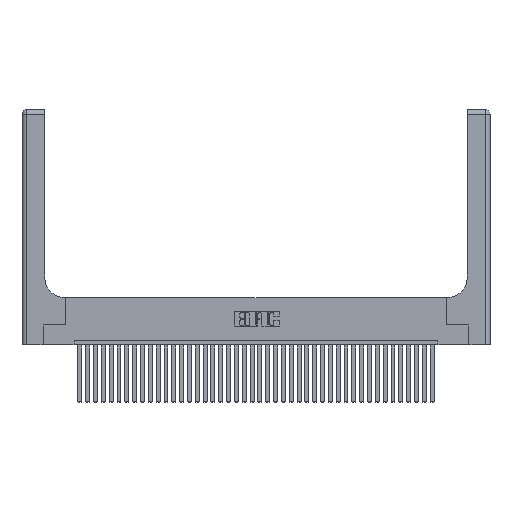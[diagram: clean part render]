
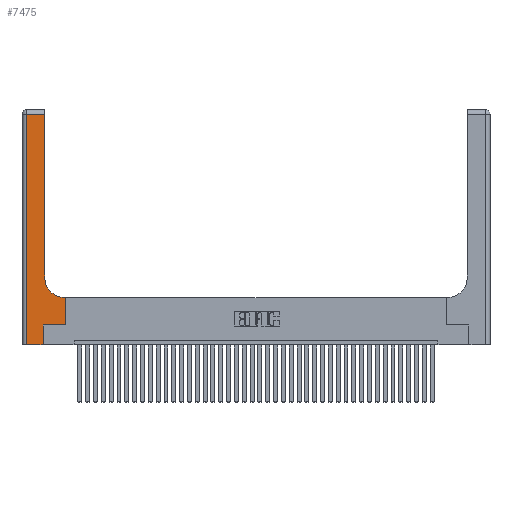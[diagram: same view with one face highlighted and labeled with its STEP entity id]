
A CAD part, top view. The second image highlights one B-rep face of the part: STEP entity #7475.
In plain terms, the highlighted planar face has unit normal (0, 0, 1).
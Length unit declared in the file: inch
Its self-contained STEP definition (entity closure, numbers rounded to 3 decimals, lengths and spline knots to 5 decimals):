
#110 = VECTOR ( 'NONE', #11667, 39.37008 ) ;
#833 = VECTOR ( 'NONE', #35096, 39.37008 ) ;
#1074 = LINE ( 'NONE', #33488, #17229 ) ;
#1376 = DIRECTION ( 'NONE',  ( -1., 0., 0. ) ) ;
#1617 = CARTESIAN_POINT ( 'NONE',  ( 0.06, 0., 0.37 ) ) ;
#1853 = LINE ( 'NONE', #7689, #833 ) ;
#2004 = ORIENTED_EDGE ( 'NONE', *, *, #32239, .T. ) ;
#2852 = ORIENTED_EDGE ( 'NONE', *, *, #15373, .T. ) ;
#4505 = DIRECTION ( 'NONE',  ( -1., 0., 0. ) ) ;
#5260 = CARTESIAN_POINT ( 'NONE',  ( 0.2915, 0.85, 0.37 ) ) ;
#5658 = EDGE_LOOP ( 'NONE', ( #2852, #28928, #32468, #20395, #30731, #34978, #31533, #2004, #23931 ) ) ;
#5990 = VERTEX_POINT ( 'NONE', #32573 ) ;
#6910 = DIRECTION ( 'NONE',  ( -1., 0., 0. ) ) ;
#7069 = DIRECTION ( 'NONE',  ( 0., 0., -1. ) ) ;
#7203 = PLANE ( 'NONE',  #17734 ) ;
#7336 = VECTOR ( 'NONE', #6910, 39.37008 ) ;
#7390 = LINE ( 'NONE', #30518, #8805 ) ;
#7475 = ADVANCED_FACE ( 'NONE', ( #32360 ), #7203, .F. ) ;
#7689 = CARTESIAN_POINT ( 'NONE',  ( 0., 0., 0.37 ) ) ;
#8541 = EDGE_CURVE ( 'NONE', #35773, #21670, #36857, .T. ) ;
#8805 = VECTOR ( 'NONE', #9416, 39.37008 ) ;
#9416 = DIRECTION ( 'NONE',  ( 0., 1., 0. ) ) ;
#10123 = VERTEX_POINT ( 'NONE', #34058 ) ;
#11398 = AXIS2_PLACEMENT_3D ( 'NONE', #24313, #18217, #30767 ) ;
#11667 = DIRECTION ( 'NONE',  ( 0., 1., 0. ) ) ;
#12252 = VERTEX_POINT ( 'NONE', #33905 ) ;
#13229 = EDGE_CURVE ( 'NONE', #32001, #12252, #24345, .T. ) ;
#13481 = CARTESIAN_POINT ( 'NONE',  ( 0.2915, 0.6, 0.37 ) ) ;
#15198 = DIRECTION ( 'NONE',  ( 0., -1., 0. ) ) ;
#15335 = CARTESIAN_POINT ( 'NONE',  ( 0.2915, 2.94, 0.37 ) ) ;
#15373 = EDGE_CURVE ( 'NONE', #31047, #32001, #35571, .T. ) ;
#15817 = CARTESIAN_POINT ( 'NONE',  ( 0.2915, 3., 0.37 ) ) ;
#17229 = VECTOR ( 'NONE', #15198, 39.37008 ) ;
#17597 = EDGE_CURVE ( 'NONE', #5990, #31047, #22143, .T. ) ;
#17734 = AXIS2_PLACEMENT_3D ( 'NONE', #22519, #7069, #1376 ) ;
#17858 = VERTEX_POINT ( 'NONE', #29990 ) ;
#18140 = CARTESIAN_POINT ( 'NONE',  ( 0., 2.94, 0.37 ) ) ;
#18217 = DIRECTION ( 'NONE',  ( 0., 0., -1. ) ) ;
#18834 = DIRECTION ( 'NONE',  ( 0., 1., 0. ) ) ;
#20100 = VERTEX_POINT ( 'NONE', #1617 ) ;
#20306 = EDGE_CURVE ( 'NONE', #21670, #10123, #37862, .T. ) ;
#20395 = ORIENTED_EDGE ( 'NONE', *, *, #34168, .T. ) ;
#21670 = VERTEX_POINT ( 'NONE', #34632 ) ;
#21705 = CARTESIAN_POINT ( 'NONE',  ( 0.269, 0.25, 0.37 ) ) ;
#22143 = CIRCLE ( 'NONE', #11398, 0.25 ) ;
#22519 = CARTESIAN_POINT ( 'NONE',  ( 0., 3., 0.37 ) ) ;
#23104 = DIRECTION ( 'NONE',  ( 1., 0., 0. ) ) ;
#23931 = ORIENTED_EDGE ( 'NONE', *, *, #17597, .T. ) ;
#24313 = CARTESIAN_POINT ( 'NONE',  ( 0.5415, 0.85, 0.37 ) ) ;
#24345 = LINE ( 'NONE', #18140, #7336 ) ;
#24432 = EDGE_CURVE ( 'NONE', #17858, #35773, #7390, .T. ) ;
#28928 = ORIENTED_EDGE ( 'NONE', *, *, #13229, .T. ) ;
#29246 = LINE ( 'NONE', #13481, #37620 ) ;
#29990 = CARTESIAN_POINT ( 'NONE',  ( 0.269, 0., 0.37 ) ) ;
#30131 = CARTESIAN_POINT ( 'NONE',  ( 0.5585, 0.25, 0.37 ) ) ;
#30518 = CARTESIAN_POINT ( 'NONE',  ( 0.269, 0., 0.37 ) ) ;
#30731 = ORIENTED_EDGE ( 'NONE', *, *, #24432, .T. ) ;
#30767 = DIRECTION ( 'NONE',  ( 1., 0., 0. ) ) ;
#31047 = VERTEX_POINT ( 'NONE', #5260 ) ;
#31533 = ORIENTED_EDGE ( 'NONE', *, *, #20306, .T. ) ;
#32001 = VERTEX_POINT ( 'NONE', #15335 ) ;
#32239 = EDGE_CURVE ( 'NONE', #10123, #5990, #29246, .T. ) ;
#32360 = FACE_OUTER_BOUND ( 'NONE', #5658, .T. ) ;
#32468 = ORIENTED_EDGE ( 'NONE', *, *, #36963, .T. ) ;
#32484 = CARTESIAN_POINT ( 'NONE',  ( 0.269, 0.25, 0.37 ) ) ;
#32573 = CARTESIAN_POINT ( 'NONE',  ( 0.5415, 0.6, 0.37 ) ) ;
#33488 = CARTESIAN_POINT ( 'NONE',  ( 0.06, 3., 0.37 ) ) ;
#33905 = CARTESIAN_POINT ( 'NONE',  ( 0.06, 2.94, 0.37 ) ) ;
#34058 = CARTESIAN_POINT ( 'NONE',  ( 0.5585, 0.6, 0.37 ) ) ;
#34168 = EDGE_CURVE ( 'NONE', #20100, #17858, #1853, .T. ) ;
#34632 = CARTESIAN_POINT ( 'NONE',  ( 0.5585, 0.25, 0.37 ) ) ;
#34978 = ORIENTED_EDGE ( 'NONE', *, *, #8541, .T. ) ;
#35094 = VECTOR ( 'NONE', #18834, 39.37008 ) ;
#35096 = DIRECTION ( 'NONE',  ( 1., 0., 0. ) ) ;
#35539 = VECTOR ( 'NONE', #23104, 39.37008 ) ;
#35571 = LINE ( 'NONE', #15817, #35094 ) ;
#35773 = VERTEX_POINT ( 'NONE', #21705 ) ;
#36857 = LINE ( 'NONE', #32484, #35539 ) ;
#36963 = EDGE_CURVE ( 'NONE', #12252, #20100, #1074, .T. ) ;
#37620 = VECTOR ( 'NONE', #4505, 39.37008 ) ;
#37862 = LINE ( 'NONE', #30131, #110 ) ;
